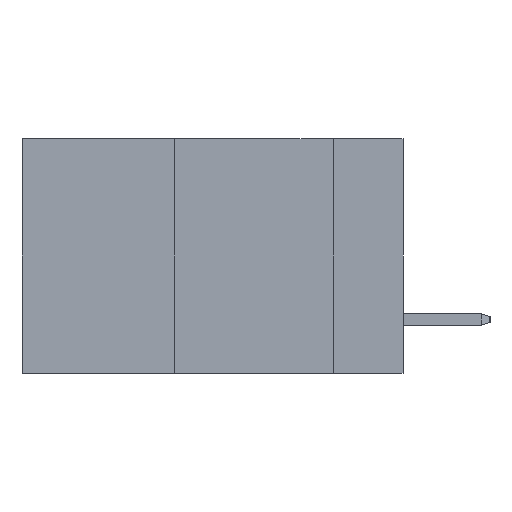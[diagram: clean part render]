
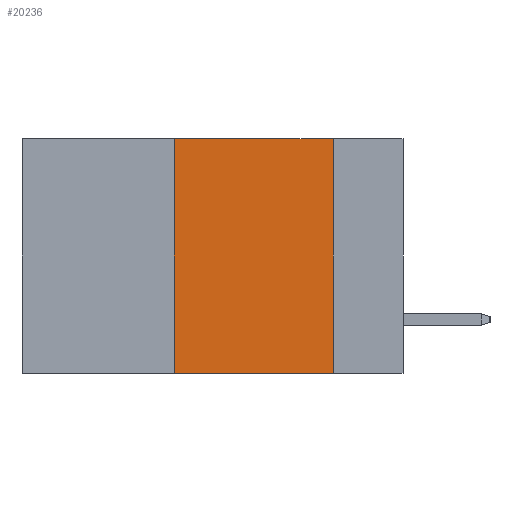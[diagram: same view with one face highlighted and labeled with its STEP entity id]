
A CAD part, left-side view. The second image highlights one B-rep face of the part: STEP entity #20236.
In plain terms, the highlighted planar face has unit normal (-1, 0, 0).
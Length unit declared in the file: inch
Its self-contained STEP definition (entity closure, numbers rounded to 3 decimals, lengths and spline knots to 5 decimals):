
#468 = CARTESIAN_POINT ( 'NONE',  ( 0., 0.6, -0.37 ) ) ;
#713 = LINE ( 'NONE', #468, #20006 ) ;
#1479 = ORIENTED_EDGE ( 'NONE', *, *, #18511, .F. ) ;
#1497 = DIRECTION ( 'NONE',  ( 1., 0., 0. ) ) ;
#1992 = CARTESIAN_POINT ( 'NONE',  ( 0., 0.6, 0. ) ) ;
#3620 = VERTEX_POINT ( 'NONE', #19970 ) ;
#3900 = EDGE_LOOP ( 'NONE', ( #18512, #6109, #1479, #22203 ) ) ;
#4088 = CARTESIAN_POINT ( 'NONE',  ( 0., 0.11, 0. ) ) ;
#5290 = FACE_OUTER_BOUND ( 'NONE', #3900, .T. ) ;
#5850 = DIRECTION ( 'NONE',  ( 0., 0., -1. ) ) ;
#5971 = LINE ( 'NONE', #4088, #15341 ) ;
#6107 = CARTESIAN_POINT ( 'NONE',  ( 0., 0.6, 0. ) ) ;
#6109 = ORIENTED_EDGE ( 'NONE', *, *, #24421, .F. ) ;
#6357 = LINE ( 'NONE', #6107, #23145 ) ;
#7619 = AXIS2_PLACEMENT_3D ( 'NONE', #1992, #1497, #11490 ) ;
#7948 = VERTEX_POINT ( 'NONE', #9832 ) ;
#8949 = VECTOR ( 'NONE', #20252, 39.37008 ) ;
#9832 = CARTESIAN_POINT ( 'NONE',  ( 0., 0.36, -0.37 ) ) ;
#10029 = DIRECTION ( 'NONE',  ( 0., -1., 0. ) ) ;
#10474 = VERTEX_POINT ( 'NONE', #23064 ) ;
#11490 = DIRECTION ( 'NONE',  ( 0., 0., -1. ) ) ;
#11605 = PLANE ( 'NONE',  #7619 ) ;
#12535 = CARTESIAN_POINT ( 'NONE',  ( 0., 0.36, 0. ) ) ;
#13838 = EDGE_CURVE ( 'NONE', #7948, #10474, #713, .T. ) ;
#13879 = DIRECTION ( 'NONE',  ( 0., -1., 0. ) ) ;
#15341 = VECTOR ( 'NONE', #5850, 39.37008 ) ;
#16567 = LINE ( 'NONE', #12535, #8949 ) ;
#18511 = EDGE_CURVE ( 'NONE', #7948, #22769, #16567, .T. ) ;
#18512 = ORIENTED_EDGE ( 'NONE', *, *, #21186, .F. ) ;
#19970 = CARTESIAN_POINT ( 'NONE',  ( 0., 0.11, 0. ) ) ;
#20006 = VECTOR ( 'NONE', #13879, 39.37008 ) ;
#20236 = ADVANCED_FACE ( 'NONE', ( #5290 ), #11605, .F. ) ;
#20252 = DIRECTION ( 'NONE',  ( 0., 0., 1. ) ) ;
#20655 = CARTESIAN_POINT ( 'NONE',  ( 0., 0.36, 0. ) ) ;
#21186 = EDGE_CURVE ( 'NONE', #3620, #10474, #5971, .T. ) ;
#22203 = ORIENTED_EDGE ( 'NONE', *, *, #13838, .T. ) ;
#22769 = VERTEX_POINT ( 'NONE', #20655 ) ;
#23064 = CARTESIAN_POINT ( 'NONE',  ( 0., 0.11, -0.37 ) ) ;
#23145 = VECTOR ( 'NONE', #10029, 39.37008 ) ;
#24421 = EDGE_CURVE ( 'NONE', #22769, #3620, #6357, .T. ) ;
